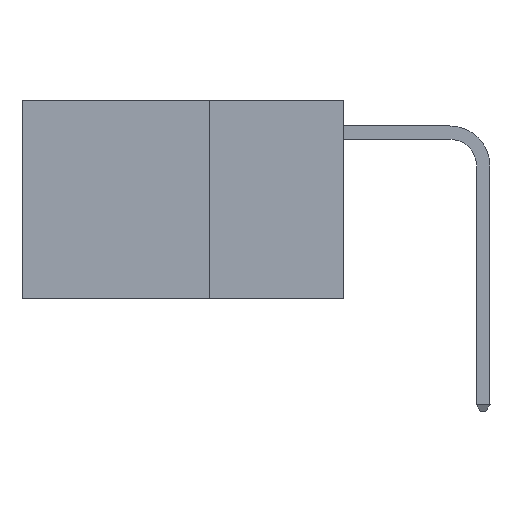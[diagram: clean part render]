
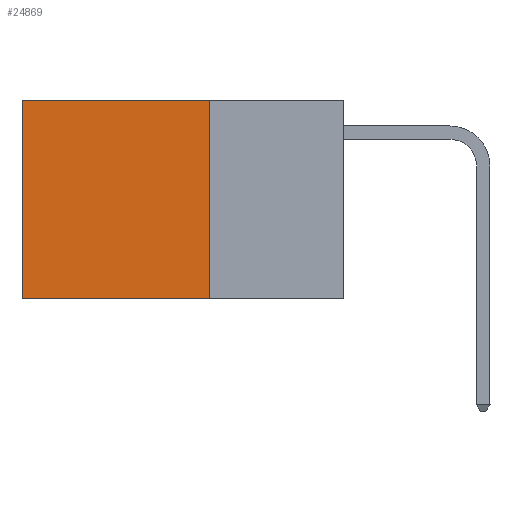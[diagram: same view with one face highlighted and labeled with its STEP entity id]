
A CAD part, left-side view. The second image highlights one B-rep face of the part: STEP entity #24869.
In plain terms, the highlighted planar face has unit normal (-1, 0, 0).
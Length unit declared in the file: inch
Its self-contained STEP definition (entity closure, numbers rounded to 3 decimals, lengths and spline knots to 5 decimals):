
#500 = VERTEX_POINT ( 'NONE', #6408 ) ;
#2194 = VECTOR ( 'NONE', #12317, 39.37008 ) ;
#2207 = ORIENTED_EDGE ( 'NONE', *, *, #23649, .F. ) ;
#3929 = LINE ( 'NONE', #18701, #13782 ) ;
#3939 = DIRECTION ( 'NONE',  ( 0., 1., 0. ) ) ;
#4084 = LINE ( 'NONE', #10205, #23813 ) ;
#4129 = LINE ( 'NONE', #10349, #2194 ) ;
#4629 = CARTESIAN_POINT ( 'NONE',  ( 0.2625, 0.25, 0. ) ) ;
#6152 = AXIS2_PLACEMENT_3D ( 'NONE', #4629, #18453, #6627 ) ;
#6408 = CARTESIAN_POINT ( 'NONE',  ( 0.2625, 0.6, 0. ) ) ;
#6627 = DIRECTION ( 'NONE',  ( 0., 0., -1. ) ) ;
#9512 = VECTOR ( 'NONE', #3939, 39.37008 ) ;
#10205 = CARTESIAN_POINT ( 'NONE',  ( 0.2625, 0.25, 0. ) ) ;
#10349 = CARTESIAN_POINT ( 'NONE',  ( 0.2625, 0.25, -0.37 ) ) ;
#10702 = VERTEX_POINT ( 'NONE', #21152 ) ;
#11054 = EDGE_LOOP ( 'NONE', ( #25580, #2207, #14396, #24167 ) ) ;
#12173 = DIRECTION ( 'NONE',  ( 0., 0., -1. ) ) ;
#12317 = DIRECTION ( 'NONE',  ( 0., 1., 0. ) ) ;
#13040 = EDGE_CURVE ( 'NONE', #500, #18608, #3929, .T. ) ;
#13236 = EDGE_CURVE ( 'NONE', #14462, #500, #14080, .T. ) ;
#13782 = VECTOR ( 'NONE', #20709, 39.37008 ) ;
#14080 = LINE ( 'NONE', #17769, #9512 ) ;
#14396 = ORIENTED_EDGE ( 'NONE', *, *, #15888, .F. ) ;
#14462 = VERTEX_POINT ( 'NONE', #21628 ) ;
#15888 = EDGE_CURVE ( 'NONE', #14462, #10702, #4084, .T. ) ;
#17769 = CARTESIAN_POINT ( 'NONE',  ( 0.2625, 0.25, 0. ) ) ;
#18453 = DIRECTION ( 'NONE',  ( 1., 0., 0. ) ) ;
#18608 = VERTEX_POINT ( 'NONE', #21883 ) ;
#18701 = CARTESIAN_POINT ( 'NONE',  ( 0.2625, 0.6, 0. ) ) ;
#20709 = DIRECTION ( 'NONE',  ( 0., 0., -1. ) ) ;
#21152 = CARTESIAN_POINT ( 'NONE',  ( 0.2625, 0.25, -0.37 ) ) ;
#21628 = CARTESIAN_POINT ( 'NONE',  ( 0.2625, 0.25, 0. ) ) ;
#21883 = CARTESIAN_POINT ( 'NONE',  ( 0.2625, 0.6, -0.37 ) ) ;
#22297 = PLANE ( 'NONE',  #6152 ) ;
#22873 = FACE_OUTER_BOUND ( 'NONE', #11054, .T. ) ;
#23649 = EDGE_CURVE ( 'NONE', #10702, #18608, #4129, .T. ) ;
#23813 = VECTOR ( 'NONE', #12173, 39.37008 ) ;
#24167 = ORIENTED_EDGE ( 'NONE', *, *, #13236, .T. ) ;
#24869 = ADVANCED_FACE ( 'NONE', ( #22873 ), #22297, .F. ) ;
#25580 = ORIENTED_EDGE ( 'NONE', *, *, #13040, .T. ) ;
